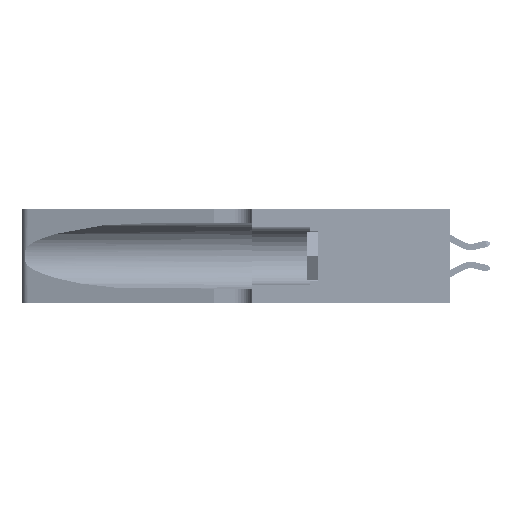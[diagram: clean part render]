
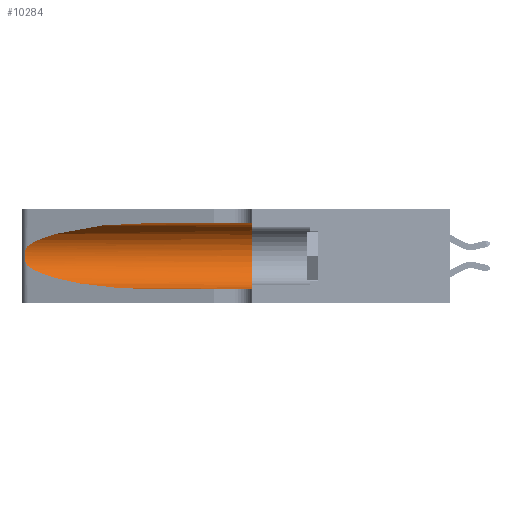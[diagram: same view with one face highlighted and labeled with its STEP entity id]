
A CAD part, left-side view. The second image highlights one B-rep face of the part: STEP entity #10284.
In plain terms, the highlighted cylindrical face has radius 3.308 mm (diameter 6.617 mm), a partial arc.
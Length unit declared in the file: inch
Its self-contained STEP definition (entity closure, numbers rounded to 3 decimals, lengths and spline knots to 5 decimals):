
#29 = EDGE_CURVE ( 'NONE', #10913, #4873, #196, .T. ) ;
#196 = LINE ( 'NONE', #36338, #9733 ) ;
#322 = DIRECTION ( 'NONE',  ( 0., -1., 0. ) ) ;
#1557 = AXIS2_PLACEMENT_3D ( 'NONE', #3842, #29049, #7459 ) ;
#2941 = CARTESIAN_POINT ( 'NONE',  ( 0.25856, 1.23593, 0.16098 ) ) ;
#3279 = CARTESIAN_POINT ( 'NONE',  ( 0.18966, 0.96281, 0.31525 ) ) ;
#3842 = CARTESIAN_POINT ( 'NONE',  ( 0.1305, 0.35, 0.185 ) ) ;
#4614 = EDGE_LOOP ( 'NONE', ( #39472, #6832, #24209, #26898, #25273, #41613 ) ) ;
#4873 = VERTEX_POINT ( 'NONE', #18904 ) ;
#6571 = CARTESIAN_POINT ( 'NONE',  ( 0.25639, 1.23186, 0.15144 ) ) ;
#6832 = ORIENTED_EDGE ( 'NONE', *, *, #23060, .T. ) ;
#7056 = AXIS2_PLACEMENT_3D ( 'NONE', #39306, #32296, #35861 ) ;
#7459 = DIRECTION ( 'NONE',  ( 0., 0., 1. ) ) ;
#8076 = CARTESIAN_POINT ( 'NONE',  ( 0.1305, 1.61858, 0.05475 ) ) ;
#8197 = CARTESIAN_POINT ( 'NONE',  ( 0.1305, 0.35, 0.05475 ) ) ;
#9161 = CARTESIAN_POINT ( 'NONE',  ( 0.25487, 1.22718, 0.22369 ) ) ;
#9733 = VECTOR ( 'NONE', #322, 39.37008 ) ;
#10014 = CARTESIAN_POINT ( 'NONE',  ( 0.25555, 1.22994, 0.2215 ) ) ;
#10181 = CARTESIAN_POINT ( 'NONE',  ( 0.25487, 1.22718, 0.14631 ) ) ;
#10284 = ADVANCED_FACE ( 'NONE', ( #20882 ), #37761, .F. ) ;
#10506 = CARTESIAN_POINT ( 'NONE',  ( 0.2373, 1.15595, 0.28018 ) ) ;
#10913 = VERTEX_POINT ( 'NONE', #21842 ) ;
#11664 = DIRECTION ( 'NONE',  ( 0., -1., 0. ) ) ;
#11815 = CARTESIAN_POINT ( 'NONE',  ( 0.18966, 0.96281, 0.05475 ) ) ;
#11965 = CARTESIAN_POINT ( 'NONE',  ( 0.1305, 0.72297, 0.05475 ) ) ;
#12969 = EDGE_CURVE ( 'NONE', #4873, #20270, #15035, .T. ) ;
#13647 = CARTESIAN_POINT ( 'NONE',  ( 0.25639, 1.23184, 0.21858 ) ) ;
#15035 = CIRCLE ( 'NONE', #1557, 0.13025 ) ;
#17105 = CARTESIAN_POINT ( 'NONE',  ( 0.25487, 1.22718, 0.22369 ) ) ;
#17252 = CARTESIAN_POINT ( 'NONE',  ( 0.25854, 1.2359, 0.20912 ) ) ;
#17683 = B_SPLINE_CURVE_WITH_KNOTS ( 'NONE', 3,
 ( #17105, #10014, #13647, #38788, #17252, #42398, #20877, #46003, #24545, #2941, #28158, #6571, #31792, #10181 ),
 .UNSPECIFIED., .F., .F.,
 ( 4, 2, 2, 2, 2, 2, 4 ),
 ( 0., 0.00027, 0.00053, 0.00107, 0.0016, 0.00187, 0.00214 ),
 .UNSPECIFIED. ) ;
#18904 = CARTESIAN_POINT ( 'NONE',  ( 0.1305, 0.35, 0.31525 ) ) ;
#20270 = VERTEX_POINT ( 'NONE', #8197 ) ;
#20877 = CARTESIAN_POINT ( 'NONE',  ( 0.26075, 1.23896, 0.19203 ) ) ;
#20882 = FACE_OUTER_BOUND ( 'NONE', #4614, .T. ) ;
#21842 = CARTESIAN_POINT ( 'NONE',  ( 0.1305, 0.72297, 0.31525 ) ) ;
#22177 = EDGE_CURVE ( 'NONE', #35052, #28193, #26107, .T. ) ;
#23060 = EDGE_CURVE ( 'NONE', #31784, #35052, #17683, .T. ) ;
#24209 = ORIENTED_EDGE ( 'NONE', *, *, #22177, .T. ) ;
#24545 = CARTESIAN_POINT ( 'NONE',  ( 0.26017, 1.23833, 0.17102 ) ) ;
#25273 = ORIENTED_EDGE ( 'NONE', *, *, #12969, .F. ) ;
#25466 = CARTESIAN_POINT ( 'NONE',  ( 0.25487, 1.22718, 0.14631 ) ) ;
#26107 =( BOUNDED_CURVE ( )  B_SPLINE_CURVE ( 3, ( #33540, #26341, #11815, #11965 ),
 .UNSPECIFIED., .F., .F. ) 
 B_SPLINE_CURVE_WITH_KNOTS ( ( 4, 4 ),
 ( 3.44316, 4.71239 ),
 .UNSPECIFIED. ) 
 CURVE ( )  GEOMETRIC_REPRESENTATION_ITEM ( )  RATIONAL_B_SPLINE_CURVE ( ( 1., 0.87, 0.87, 1. ) ) 
 REPRESENTATION_ITEM ( '' )  );
#26341 = CARTESIAN_POINT ( 'NONE',  ( 0.2373, 1.15595, 0.08982 ) ) ;
#26798 = EDGE_CURVE ( 'NONE', #28193, #20270, #26886, .T. ) ;
#26886 = LINE ( 'NONE', #8076, #44828 ) ;
#26898 = ORIENTED_EDGE ( 'NONE', *, *, #26798, .T. ) ;
#28158 = CARTESIAN_POINT ( 'NONE',  ( 0.25789, 1.23486, 0.15765 ) ) ;
#28193 = VERTEX_POINT ( 'NONE', #33781 ) ;
#28492 = CARTESIAN_POINT ( 'NONE',  ( 0.1305, 0.72297, 0.31525 ) ) ;
#29049 = DIRECTION ( 'NONE',  ( 0., 1., 0. ) ) ;
#31007 =( BOUNDED_CURVE ( )  B_SPLINE_CURVE ( 3, ( #28492, #3279, #10506, #35681 ),
 .UNSPECIFIED., .F., .F. ) 
 B_SPLINE_CURVE_WITH_KNOTS ( ( 4, 4 ),
 ( 1.5708, 2.84003 ),
 .UNSPECIFIED. ) 
 CURVE ( )  GEOMETRIC_REPRESENTATION_ITEM ( )  RATIONAL_B_SPLINE_CURVE ( ( 1., 0.87, 0.87, 1. ) ) 
 REPRESENTATION_ITEM ( '' )  );
#31784 = VERTEX_POINT ( 'NONE', #9161 ) ;
#31792 = CARTESIAN_POINT ( 'NONE',  ( 0.25555, 1.22993, 0.14849 ) ) ;
#32296 = DIRECTION ( 'NONE',  ( 0., -1., 0. ) ) ;
#32588 = EDGE_CURVE ( 'NONE', #10913, #31784, #31007, .T. ) ;
#33540 = CARTESIAN_POINT ( 'NONE',  ( 0.25487, 1.22718, 0.14631 ) ) ;
#33781 = CARTESIAN_POINT ( 'NONE',  ( 0.1305, 0.72297, 0.05475 ) ) ;
#35052 = VERTEX_POINT ( 'NONE', #25466 ) ;
#35681 = CARTESIAN_POINT ( 'NONE',  ( 0.25487, 1.22718, 0.22369 ) ) ;
#35861 = DIRECTION ( 'NONE',  ( 0., 0., -1. ) ) ;
#36338 = CARTESIAN_POINT ( 'NONE',  ( 0.1305, 1.61858, 0.31525 ) ) ;
#37761 = CYLINDRICAL_SURFACE ( 'NONE', #7056, 0.13025 ) ;
#38788 = CARTESIAN_POINT ( 'NONE',  ( 0.25787, 1.23484, 0.2124 ) ) ;
#39306 = CARTESIAN_POINT ( 'NONE',  ( 0.1305, 1.61858, 0.185 ) ) ;
#39472 = ORIENTED_EDGE ( 'NONE', *, *, #32588, .T. ) ;
#41613 = ORIENTED_EDGE ( 'NONE', *, *, #29, .F. ) ;
#42398 = CARTESIAN_POINT ( 'NONE',  ( 0.26018, 1.23835, 0.19895 ) ) ;
#44828 = VECTOR ( 'NONE', #11664, 39.37008 ) ;
#46003 = CARTESIAN_POINT ( 'NONE',  ( 0.26075, 1.23896, 0.178 ) ) ;
